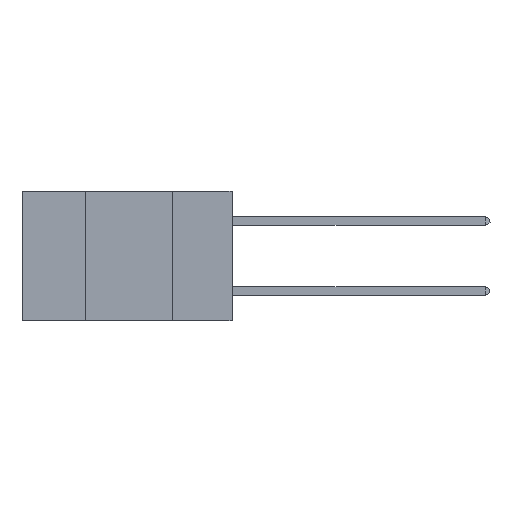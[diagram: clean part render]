
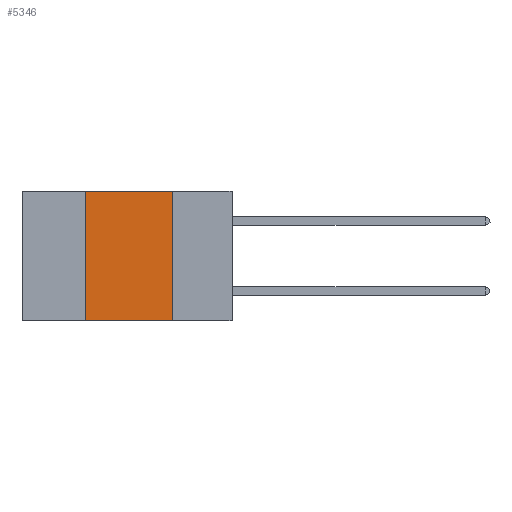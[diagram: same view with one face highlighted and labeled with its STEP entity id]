
A CAD part, left-side view. The second image highlights one B-rep face of the part: STEP entity #5346.
In plain terms, the highlighted planar face has unit normal (-1, 0, 0).
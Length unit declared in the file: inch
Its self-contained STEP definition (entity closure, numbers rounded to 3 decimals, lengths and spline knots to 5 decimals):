
#318 = EDGE_CURVE ( 'NONE', #12660, #10687, #6006, .T. ) ;
#428 = DIRECTION ( 'NONE',  ( 0., 0., -1. ) ) ;
#597 = VERTEX_POINT ( 'NONE', #13881 ) ;
#1193 = EDGE_LOOP ( 'NONE', ( #1248, #8199, #3917, #4459 ) ) ;
#1212 = LINE ( 'NONE', #13521, #12450 ) ;
#1248 = ORIENTED_EDGE ( 'NONE', *, *, #6740, .F. ) ;
#1568 = CARTESIAN_POINT ( 'NONE',  ( 0., 0.6, 0. ) ) ;
#2040 = VECTOR ( 'NONE', #12770, 39.37008 ) ;
#2045 = DIRECTION ( 'NONE',  ( 0., 0., -1. ) ) ;
#3115 = CARTESIAN_POINT ( 'NONE',  ( 0., 0.17, 0. ) ) ;
#3917 = ORIENTED_EDGE ( 'NONE', *, *, #12452, .F. ) ;
#4114 = CARTESIAN_POINT ( 'NONE',  ( 0., 0.42, 0. ) ) ;
#4325 = CARTESIAN_POINT ( 'NONE',  ( 0., 0.6, 0. ) ) ;
#4459 = ORIENTED_EDGE ( 'NONE', *, *, #12380, .T. ) ;
#5119 = CARTESIAN_POINT ( 'NONE',  ( 0., 0.42, -0.37 ) ) ;
#5346 = ADVANCED_FACE ( 'NONE', ( #5820 ), #9756, .F. ) ;
#5784 = DIRECTION ( 'NONE',  ( 0., -1., 0. ) ) ;
#5820 = FACE_OUTER_BOUND ( 'NONE', #1193, .T. ) ;
#6006 = LINE ( 'NONE', #1568, #10428 ) ;
#6221 = VERTEX_POINT ( 'NONE', #5119 ) ;
#6534 = DIRECTION ( 'NONE',  ( 1., 0., 0. ) ) ;
#6740 = EDGE_CURVE ( 'NONE', #10687, #597, #13086, .T. ) ;
#7398 = CARTESIAN_POINT ( 'NONE',  ( 0., 0.17, 0. ) ) ;
#7485 = CARTESIAN_POINT ( 'NONE',  ( 0., 0.42, 0. ) ) ;
#8199 = ORIENTED_EDGE ( 'NONE', *, *, #318, .F. ) ;
#8881 = LINE ( 'NONE', #4114, #2040 ) ;
#9756 = PLANE ( 'NONE',  #10828 ) ;
#10355 = VECTOR ( 'NONE', #428, 39.37008 ) ;
#10428 = VECTOR ( 'NONE', #5784, 39.37008 ) ;
#10687 = VERTEX_POINT ( 'NONE', #7398 ) ;
#10828 = AXIS2_PLACEMENT_3D ( 'NONE', #4325, #6534, #2045 ) ;
#12267 = DIRECTION ( 'NONE',  ( 0., -1., 0. ) ) ;
#12380 = EDGE_CURVE ( 'NONE', #6221, #597, #1212, .T. ) ;
#12450 = VECTOR ( 'NONE', #12267, 39.37008 ) ;
#12452 = EDGE_CURVE ( 'NONE', #6221, #12660, #8881, .T. ) ;
#12660 = VERTEX_POINT ( 'NONE', #7485 ) ;
#12770 = DIRECTION ( 'NONE',  ( 0., 0., 1. ) ) ;
#13086 = LINE ( 'NONE', #3115, #10355 ) ;
#13521 = CARTESIAN_POINT ( 'NONE',  ( 0., 0.6, -0.37 ) ) ;
#13881 = CARTESIAN_POINT ( 'NONE',  ( 0., 0.17, -0.37 ) ) ;
